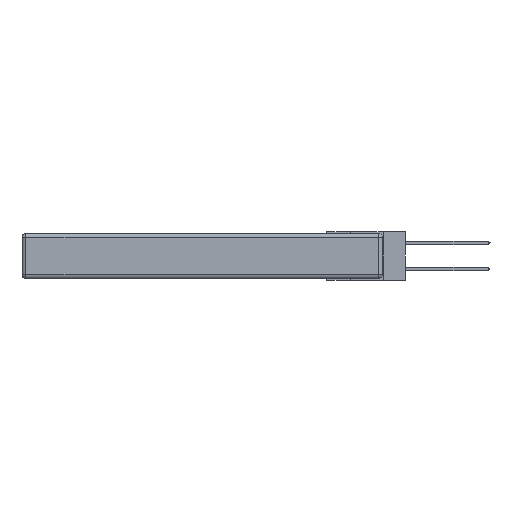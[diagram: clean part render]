
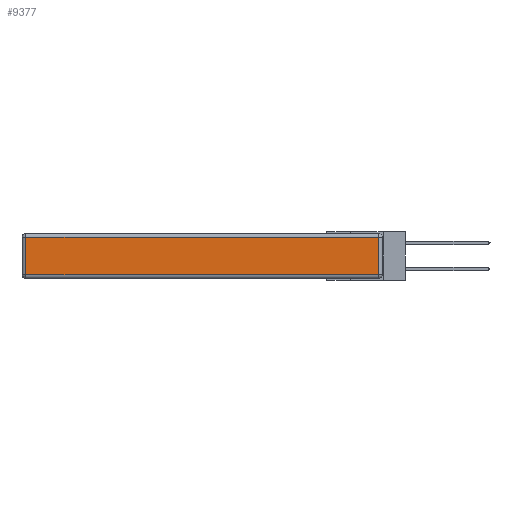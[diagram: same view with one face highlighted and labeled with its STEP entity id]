
A CAD part, left-side view. The second image highlights one B-rep face of the part: STEP entity #9377.
In plain terms, the highlighted planar face has unit normal (-1, 0, 0).
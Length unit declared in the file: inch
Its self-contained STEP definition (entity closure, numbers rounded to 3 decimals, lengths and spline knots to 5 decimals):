
#339 = VECTOR ( 'NONE', #7390, 39.37008 ) ;
#1087 = LINE ( 'NONE', #10150, #1238 ) ;
#1238 = VECTOR ( 'NONE', #12089, 39.37008 ) ;
#1249 = FACE_OUTER_BOUND ( 'NONE', #11889, .T. ) ;
#1473 = VERTEX_POINT ( 'NONE', #8130 ) ;
#2550 = DIRECTION ( 'NONE',  ( 0., -1., 0. ) ) ;
#2809 = CARTESIAN_POINT ( 'NONE',  ( 0., 2.72, -0.03 ) ) ;
#2941 = ORIENTED_EDGE ( 'NONE', *, *, #9565, .T. ) ;
#3270 = PLANE ( 'NONE',  #5553 ) ;
#3317 = DIRECTION ( 'NONE',  ( 0., 0., 1. ) ) ;
#3447 = LINE ( 'NONE', #8526, #339 ) ;
#3557 = VERTEX_POINT ( 'NONE', #2809 ) ;
#3724 = VERTEX_POINT ( 'NONE', #5314 ) ;
#3856 = ORIENTED_EDGE ( 'NONE', *, *, #4405, .T. ) ;
#4194 = VECTOR ( 'NONE', #2550, 39.37008 ) ;
#4405 = EDGE_CURVE ( 'NONE', #3557, #1473, #3447, .T. ) ;
#5314 = CARTESIAN_POINT ( 'NONE',  ( 0., 0.03, -0.313 ) ) ;
#5415 = ORIENTED_EDGE ( 'NONE', *, *, #10429, .T. ) ;
#5553 = AXIS2_PLACEMENT_3D ( 'NONE', #10247, #9275, #3317 ) ;
#6850 = LINE ( 'NONE', #7341, #4194 ) ;
#6892 = LINE ( 'NONE', #12577, #8913 ) ;
#6972 = VERTEX_POINT ( 'NONE', #10258 ) ;
#7058 = ORIENTED_EDGE ( 'NONE', *, *, #9429, .T. ) ;
#7341 = CARTESIAN_POINT ( 'NONE',  ( 0., 0., -0.313 ) ) ;
#7390 = DIRECTION ( 'NONE',  ( 0., 0., -1. ) ) ;
#8130 = CARTESIAN_POINT ( 'NONE',  ( 0., 2.72, -0.313 ) ) ;
#8526 = CARTESIAN_POINT ( 'NONE',  ( 0., 2.72, -0.343 ) ) ;
#8913 = VECTOR ( 'NONE', #9633, 39.37008 ) ;
#9275 = DIRECTION ( 'NONE',  ( -1., 0., 0. ) ) ;
#9377 = ADVANCED_FACE ( 'NONE', ( #1249 ), #3270, .T. ) ;
#9429 = EDGE_CURVE ( 'NONE', #6972, #3557, #6892, .T. ) ;
#9565 = EDGE_CURVE ( 'NONE', #3724, #6972, #1087, .T. ) ;
#9633 = DIRECTION ( 'NONE',  ( 0., 1., 0. ) ) ;
#10150 = CARTESIAN_POINT ( 'NONE',  ( 0., 0.03, -0.343 ) ) ;
#10247 = CARTESIAN_POINT ( 'NONE',  ( 0., 0., -0.343 ) ) ;
#10258 = CARTESIAN_POINT ( 'NONE',  ( 0., 0.03, -0.03 ) ) ;
#10429 = EDGE_CURVE ( 'NONE', #1473, #3724, #6850, .T. ) ;
#11889 = EDGE_LOOP ( 'NONE', ( #5415, #2941, #7058, #3856 ) ) ;
#12089 = DIRECTION ( 'NONE',  ( 0., 0., 1. ) ) ;
#12577 = CARTESIAN_POINT ( 'NONE',  ( 0., 2.75, -0.03 ) ) ;
